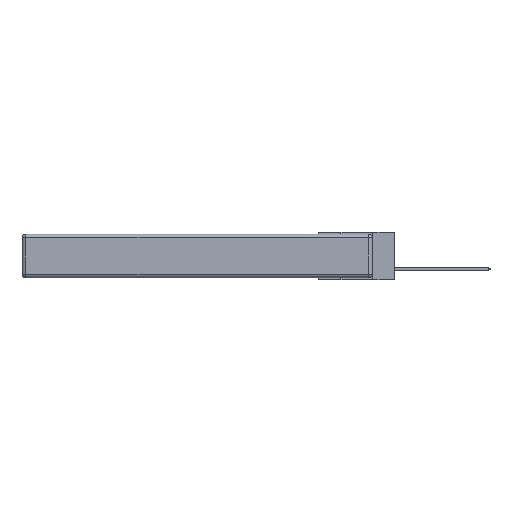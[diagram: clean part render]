
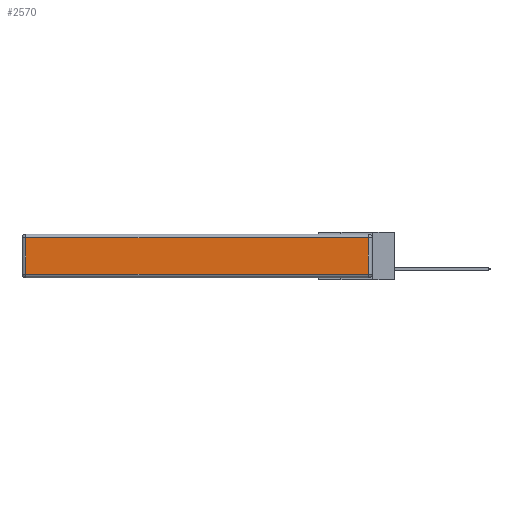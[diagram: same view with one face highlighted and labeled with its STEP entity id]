
A CAD part, left-side view. The second image highlights one B-rep face of the part: STEP entity #2570.
In plain terms, the highlighted planar face has unit normal (-1, 0, 0).
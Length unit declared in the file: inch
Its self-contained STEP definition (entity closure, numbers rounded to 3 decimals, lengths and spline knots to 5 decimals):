
#44 = CARTESIAN_POINT ( 'NONE',  ( 0., 0.03, -0.313 ) ) ;
#191 = VECTOR ( 'NONE', #3999, 39.37008 ) ;
#1054 = CARTESIAN_POINT ( 'NONE',  ( 0., 0.03, -0.343 ) ) ;
#1190 = CARTESIAN_POINT ( 'NONE',  ( 0., 2.75, -0.03 ) ) ;
#1854 = ORIENTED_EDGE ( 'NONE', *, *, #5416, .T. ) ;
#1873 = ORIENTED_EDGE ( 'NONE', *, *, #3406, .T. ) ;
#2049 = VECTOR ( 'NONE', #11400, 39.37008 ) ;
#2140 = ORIENTED_EDGE ( 'NONE', *, *, #8800, .T. ) ;
#2279 = CARTESIAN_POINT ( 'NONE',  ( 0., 2.72, -0.313 ) ) ;
#2454 = AXIS2_PLACEMENT_3D ( 'NONE', #5672, #5718, #11466 ) ;
#2461 = ORIENTED_EDGE ( 'NONE', *, *, #11863, .T. ) ;
#2570 = ADVANCED_FACE ( 'NONE', ( #3403 ), #5641, .T. ) ;
#3164 = LINE ( 'NONE', #8838, #191 ) ;
#3196 = VECTOR ( 'NONE', #10159, 39.37008 ) ;
#3403 = FACE_OUTER_BOUND ( 'NONE', #9415, .T. ) ;
#3406 = EDGE_CURVE ( 'NONE', #4222, #6761, #11388, .T. ) ;
#3483 = VERTEX_POINT ( 'NONE', #44 ) ;
#3999 = DIRECTION ( 'NONE',  ( 0., -1., 0. ) ) ;
#4222 = VERTEX_POINT ( 'NONE', #6593 ) ;
#4832 = CARTESIAN_POINT ( 'NONE',  ( 0., 0.03, -0.03 ) ) ;
#5416 = EDGE_CURVE ( 'NONE', #6761, #3483, #3164, .T. ) ;
#5641 = PLANE ( 'NONE',  #2454 ) ;
#5672 = CARTESIAN_POINT ( 'NONE',  ( 0., 0., -0.343 ) ) ;
#5718 = DIRECTION ( 'NONE',  ( -1., 0., 0. ) ) ;
#5759 = LINE ( 'NONE', #1190, #3196 ) ;
#5786 = VECTOR ( 'NONE', #11650, 39.37008 ) ;
#6593 = CARTESIAN_POINT ( 'NONE',  ( 0., 2.72, -0.03 ) ) ;
#6761 = VERTEX_POINT ( 'NONE', #2279 ) ;
#8460 = CARTESIAN_POINT ( 'NONE',  ( 0., 2.72, -0.343 ) ) ;
#8800 = EDGE_CURVE ( 'NONE', #3483, #9152, #9875, .T. ) ;
#8838 = CARTESIAN_POINT ( 'NONE',  ( 0., 0., -0.313 ) ) ;
#9152 = VERTEX_POINT ( 'NONE', #4832 ) ;
#9415 = EDGE_LOOP ( 'NONE', ( #1854, #2140, #2461, #1873 ) ) ;
#9875 = LINE ( 'NONE', #1054, #5786 ) ;
#10159 = DIRECTION ( 'NONE',  ( 0., 1., 0. ) ) ;
#11388 = LINE ( 'NONE', #8460, #2049 ) ;
#11400 = DIRECTION ( 'NONE',  ( 0., 0., -1. ) ) ;
#11466 = DIRECTION ( 'NONE',  ( 0., 0., 1. ) ) ;
#11650 = DIRECTION ( 'NONE',  ( 0., 0., 1. ) ) ;
#11863 = EDGE_CURVE ( 'NONE', #9152, #4222, #5759, .T. ) ;
